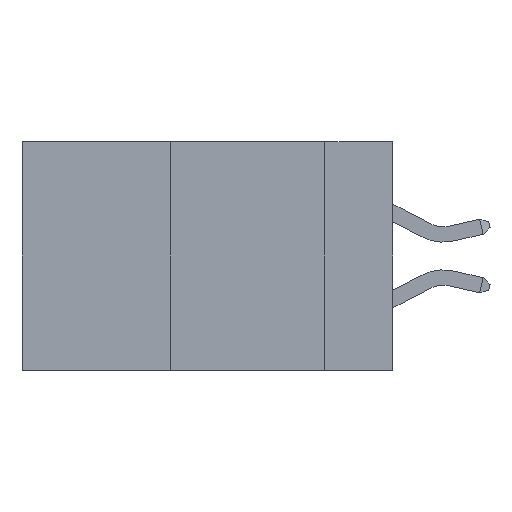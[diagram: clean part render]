
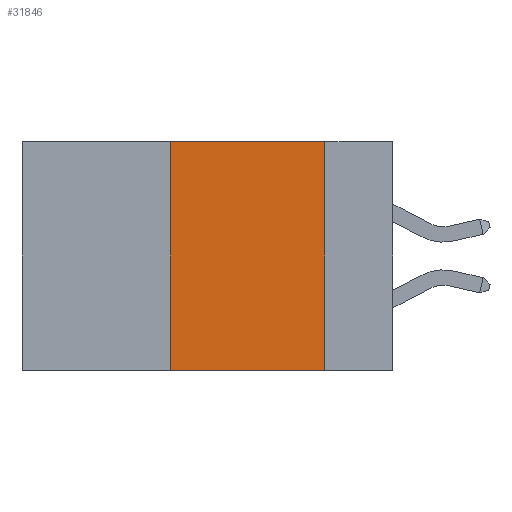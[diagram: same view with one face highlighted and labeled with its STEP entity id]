
A CAD part, left-side view. The second image highlights one B-rep face of the part: STEP entity #31846.
In plain terms, the highlighted planar face has unit normal (-1, 0, 0).
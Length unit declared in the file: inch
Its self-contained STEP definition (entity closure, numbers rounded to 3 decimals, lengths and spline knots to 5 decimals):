
#933 = LINE ( 'NONE', #15245, #16695 ) ;
#940 = VECTOR ( 'NONE', #35457, 39.37008 ) ;
#2263 = CARTESIAN_POINT ( 'NONE',  ( 0., 0.11, -0.37 ) ) ;
#2956 = LINE ( 'NONE', #33459, #18721 ) ;
#4107 = CARTESIAN_POINT ( 'NONE',  ( 0., 0.11, 0. ) ) ;
#6721 = CARTESIAN_POINT ( 'NONE',  ( 0., 0.36, 0. ) ) ;
#6735 = CARTESIAN_POINT ( 'NONE',  ( 0., 0.36, -0.37 ) ) ;
#7393 = CARTESIAN_POINT ( 'NONE',  ( 0., 0.36, 0. ) ) ;
#7870 = PLANE ( 'NONE',  #14587 ) ;
#8109 = EDGE_CURVE ( 'NONE', #20466, #30787, #2956, .T. ) ;
#8396 = EDGE_CURVE ( 'NONE', #22430, #20466, #17221, .T. ) ;
#9267 = ORIENTED_EDGE ( 'NONE', *, *, #32245, .F. ) ;
#9300 = LINE ( 'NONE', #4107, #940 ) ;
#12165 = CARTESIAN_POINT ( 'NONE',  ( 0., 0.11, 0. ) ) ;
#14145 = DIRECTION ( 'NONE',  ( 0., 0., -1. ) ) ;
#14201 = EDGE_CURVE ( 'NONE', #22430, #26262, #933, .T. ) ;
#14587 = AXIS2_PLACEMENT_3D ( 'NONE', #29792, #32916, #14145 ) ;
#15206 = VECTOR ( 'NONE', #19239, 39.37008 ) ;
#15245 = CARTESIAN_POINT ( 'NONE',  ( 0., 0.6, -0.37 ) ) ;
#16695 = VECTOR ( 'NONE', #37090, 39.37008 ) ;
#17221 = LINE ( 'NONE', #6721, #15206 ) ;
#18721 = VECTOR ( 'NONE', #36551, 39.37008 ) ;
#19239 = DIRECTION ( 'NONE',  ( 0., 0., 1. ) ) ;
#20110 = ORIENTED_EDGE ( 'NONE', *, *, #14201, .T. ) ;
#20146 = ORIENTED_EDGE ( 'NONE', *, *, #8396, .F. ) ;
#20466 = VERTEX_POINT ( 'NONE', #7393 ) ;
#22430 = VERTEX_POINT ( 'NONE', #6735 ) ;
#26262 = VERTEX_POINT ( 'NONE', #2263 ) ;
#29792 = CARTESIAN_POINT ( 'NONE',  ( 0., 0.6, 0. ) ) ;
#30180 = ORIENTED_EDGE ( 'NONE', *, *, #8109, .F. ) ;
#30787 = VERTEX_POINT ( 'NONE', #12165 ) ;
#31407 = FACE_OUTER_BOUND ( 'NONE', #39004, .T. ) ;
#31846 = ADVANCED_FACE ( 'NONE', ( #31407 ), #7870, .F. ) ;
#32245 = EDGE_CURVE ( 'NONE', #30787, #26262, #9300, .T. ) ;
#32916 = DIRECTION ( 'NONE',  ( 1., 0., 0. ) ) ;
#33459 = CARTESIAN_POINT ( 'NONE',  ( 0., 0.6, 0. ) ) ;
#35457 = DIRECTION ( 'NONE',  ( 0., 0., -1. ) ) ;
#36551 = DIRECTION ( 'NONE',  ( 0., -1., 0. ) ) ;
#37090 = DIRECTION ( 'NONE',  ( 0., -1., 0. ) ) ;
#39004 = EDGE_LOOP ( 'NONE', ( #9267, #30180, #20146, #20110 ) ) ;
